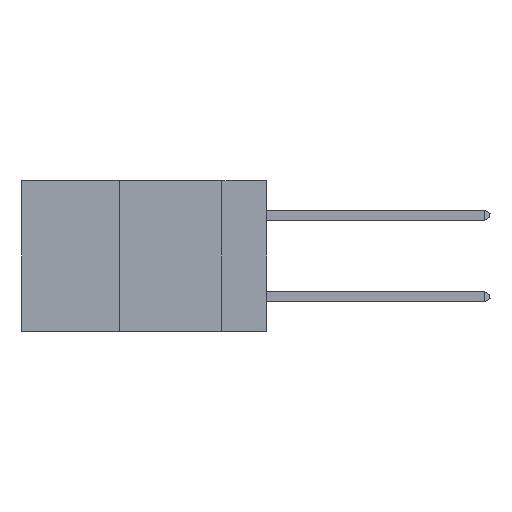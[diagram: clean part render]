
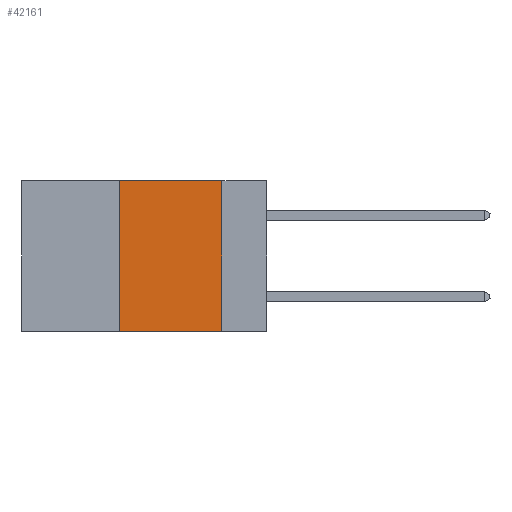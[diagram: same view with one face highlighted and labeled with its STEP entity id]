
A CAD part, left-side view. The second image highlights one B-rep face of the part: STEP entity #42161.
In plain terms, the highlighted planar face has unit normal (-1, 0, 0).
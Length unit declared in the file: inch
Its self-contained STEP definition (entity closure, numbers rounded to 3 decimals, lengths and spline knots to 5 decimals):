
#315 = VERTEX_POINT ( 'NONE', #26373 ) ;
#593 = ORIENTED_EDGE ( 'NONE', *, *, #3101, .F. ) ;
#2283 = EDGE_CURVE ( 'NONE', #38398, #25044, #47161, .T. ) ;
#2771 = LINE ( 'NONE', #31591, #21363 ) ;
#2973 = VECTOR ( 'NONE', #4824, 39.37008 ) ;
#3054 = CARTESIAN_POINT ( 'NONE',  ( 0., 0.6, 0. ) ) ;
#3101 = EDGE_CURVE ( 'NONE', #315, #25659, #24000, .T. ) ;
#4141 = LINE ( 'NONE', #23311, #2973 ) ;
#4824 = DIRECTION ( 'NONE',  ( 0., -1., 0. ) ) ;
#7625 = CARTESIAN_POINT ( 'NONE',  ( 0., 0.36, 0. ) ) ;
#9489 = EDGE_LOOP ( 'NONE', ( #593, #42579, #27425, #16791 ) ) ;
#10651 = PLANE ( 'NONE',  #22641 ) ;
#14406 = DIRECTION ( 'NONE',  ( 0., 0., -1. ) ) ;
#16791 = ORIENTED_EDGE ( 'NONE', *, *, #38780, .T. ) ;
#18196 = FACE_OUTER_BOUND ( 'NONE', #9489, .T. ) ;
#21363 = VECTOR ( 'NONE', #35196, 39.37008 ) ;
#22641 = AXIS2_PLACEMENT_3D ( 'NONE', #3054, #36077, #14406 ) ;
#23311 = CARTESIAN_POINT ( 'NONE',  ( 0., 0.6, 0. ) ) ;
#24000 = LINE ( 'NONE', #31274, #32449 ) ;
#25044 = VERTEX_POINT ( 'NONE', #29385 ) ;
#25659 = VERTEX_POINT ( 'NONE', #38314 ) ;
#25956 = CARTESIAN_POINT ( 'NONE',  ( 0., 0.36, -0.37 ) ) ;
#26373 = CARTESIAN_POINT ( 'NONE',  ( 0., 0.11, 0. ) ) ;
#27425 = ORIENTED_EDGE ( 'NONE', *, *, #2283, .F. ) ;
#28010 = VECTOR ( 'NONE', #43920, 39.37008 ) ;
#29385 = CARTESIAN_POINT ( 'NONE',  ( 0., 0.36, 0. ) ) ;
#31274 = CARTESIAN_POINT ( 'NONE',  ( 0., 0.11, 0. ) ) ;
#31591 = CARTESIAN_POINT ( 'NONE',  ( 0., 0.6, -0.37 ) ) ;
#32449 = VECTOR ( 'NONE', #42110, 39.37008 ) ;
#35196 = DIRECTION ( 'NONE',  ( 0., -1., 0. ) ) ;
#36077 = DIRECTION ( 'NONE',  ( 1., 0., 0. ) ) ;
#38314 = CARTESIAN_POINT ( 'NONE',  ( 0., 0.11, -0.37 ) ) ;
#38398 = VERTEX_POINT ( 'NONE', #25956 ) ;
#38780 = EDGE_CURVE ( 'NONE', #38398, #25659, #2771, .T. ) ;
#42110 = DIRECTION ( 'NONE',  ( 0., 0., -1. ) ) ;
#42161 = ADVANCED_FACE ( 'NONE', ( #18196 ), #10651, .F. ) ;
#42493 = EDGE_CURVE ( 'NONE', #25044, #315, #4141, .T. ) ;
#42579 = ORIENTED_EDGE ( 'NONE', *, *, #42493, .F. ) ;
#43920 = DIRECTION ( 'NONE',  ( 0., 0., 1. ) ) ;
#47161 = LINE ( 'NONE', #7625, #28010 ) ;
